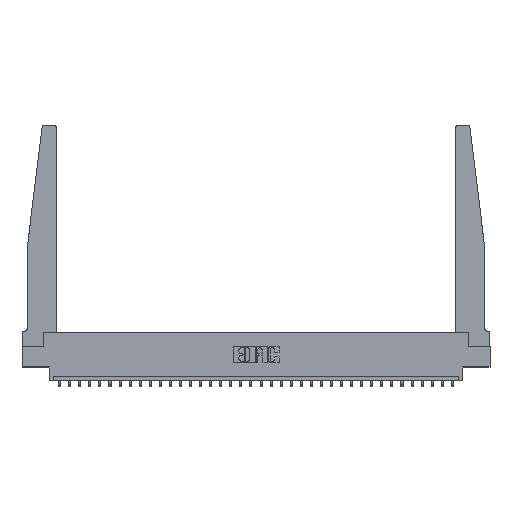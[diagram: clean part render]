
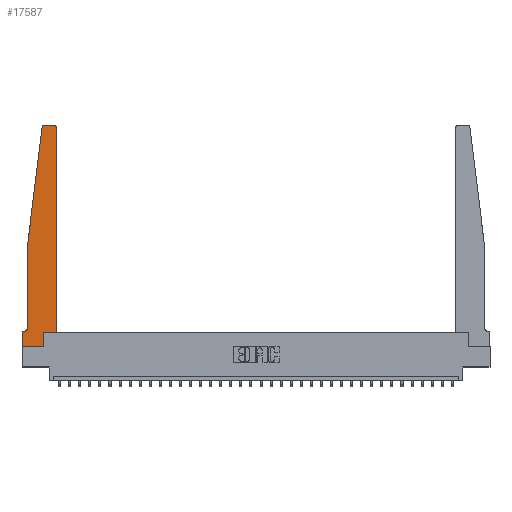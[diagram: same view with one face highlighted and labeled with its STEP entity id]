
A CAD part, top view. The second image highlights one B-rep face of the part: STEP entity #17587.
In plain terms, the highlighted planar face has unit normal (0, 0, 1).
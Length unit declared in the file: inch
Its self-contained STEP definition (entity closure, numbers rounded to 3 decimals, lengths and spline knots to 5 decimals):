
#184 = LINE ( 'NONE', #27953, #18059 ) ;
#449 = VERTEX_POINT ( 'NONE', #13266 ) ;
#829 = LINE ( 'NONE', #26259, #12484 ) ;
#838 = CARTESIAN_POINT ( 'NONE',  ( 0.065, 1.25, 0.37 ) ) ;
#891 = CARTESIAN_POINT ( 'NONE',  ( 0.015, 0.2375, 0.37 ) ) ;
#1064 = EDGE_CURVE ( 'NONE', #24890, #20575, #15991, .T. ) ;
#1639 = EDGE_CURVE ( 'NONE', #25553, #26862, #17793, .T. ) ;
#1851 = ORIENTED_EDGE ( 'NONE', *, *, #1064, .T. ) ;
#2342 = CARTESIAN_POINT ( 'NONE',  ( 0.015, 0.1875, 0.37 ) ) ;
#2371 = LINE ( 'NONE', #28194, #14041 ) ;
#2573 = DIRECTION ( 'NONE',  ( 1., 0., 0. ) ) ;
#2595 = CARTESIAN_POINT ( 'NONE',  ( 0., 0., 0.37 ) ) ;
#2944 = PLANE ( 'NONE',  #10477 ) ;
#3221 = DIRECTION ( 'NONE',  ( -1., 0., 0. ) ) ;
#3519 = VERTEX_POINT ( 'NONE', #17491 ) ;
#3600 = ORIENTED_EDGE ( 'NONE', *, *, #22285, .T. ) ;
#3821 = ORIENTED_EDGE ( 'NONE', *, *, #8251, .T. ) ;
#4082 = VECTOR ( 'NONE', #27996, 39.37008 ) ;
#4531 = LINE ( 'NONE', #6041, #16272 ) ;
#4697 = EDGE_CURVE ( 'NONE', #26949, #24890, #27327, .T. ) ;
#5114 = VERTEX_POINT ( 'NONE', #7011 ) ;
#5982 = DIRECTION ( 'NONE',  ( 0., 0., 1. ) ) ;
#6041 = CARTESIAN_POINT ( 'NONE',  ( 0.425, 0.18, 0.37 ) ) ;
#6273 = EDGE_CURVE ( 'NONE', #3519, #15491, #16355, .T. ) ;
#6381 = VERTEX_POINT ( 'NONE', #2595 ) ;
#6476 = CARTESIAN_POINT ( 'NONE',  ( 0.065, 0.2375, 0.37 ) ) ;
#6590 = ORIENTED_EDGE ( 'NONE', *, *, #24447, .T. ) ;
#6827 = AXIS2_PLACEMENT_3D ( 'NONE', #20009, #5982, #22331 ) ;
#7011 = CARTESIAN_POINT ( 'NONE',  ( 0.2605, 0., 0.37 ) ) ;
#8229 = ORIENTED_EDGE ( 'NONE', *, *, #28658, .T. ) ;
#8251 = EDGE_CURVE ( 'NONE', #5114, #449, #184, .T. ) ;
#8418 = DIRECTION ( 'NONE',  ( 0., 1., 0. ) ) ;
#8603 = ORIENTED_EDGE ( 'NONE', *, *, #10242, .T. ) ;
#8953 = CARTESIAN_POINT ( 'NONE',  ( 0., 0., 0.37 ) ) ;
#9014 = VECTOR ( 'NONE', #10866, 39.37008 ) ;
#9491 = CARTESIAN_POINT ( 'NONE',  ( 0., 0., 0.37 ) ) ;
#10206 = VERTEX_POINT ( 'NONE', #21589 ) ;
#10242 = EDGE_CURVE ( 'NONE', #15491, #10206, #16654, .T. ) ;
#10423 = EDGE_CURVE ( 'NONE', #19759, #25553, #4531, .T. ) ;
#10459 = CARTESIAN_POINT ( 'NONE',  ( 0.425, 2.72, 0.37 ) ) ;
#10477 = AXIS2_PLACEMENT_3D ( 'NONE', #26213, #12312, #28528 ) ;
#10866 = DIRECTION ( 'NONE',  ( -1., 0., 0. ) ) ;
#12312 = DIRECTION ( 'NONE',  ( 0., 0., 1. ) ) ;
#12484 = VECTOR ( 'NONE', #14592, 39.37008 ) ;
#13266 = CARTESIAN_POINT ( 'NONE',  ( 0.2605, 0.18, 0.37 ) ) ;
#13816 = DIRECTION ( 'NONE',  ( 0., 0., 1. ) ) ;
#14041 = VECTOR ( 'NONE', #18997, 39.37008 ) ;
#14592 = DIRECTION ( 'NONE',  ( 1., 0., 0. ) ) ;
#15175 = VECTOR ( 'NONE', #19484, 39.37008 ) ;
#15187 = VECTOR ( 'NONE', #2573, 39.37008 ) ;
#15491 = VERTEX_POINT ( 'NONE', #16072 ) ;
#15991 = LINE ( 'NONE', #22467, #9014 ) ;
#16072 = CARTESIAN_POINT ( 'NONE',  ( 0.24675, 2.72367, 0.37 ) ) ;
#16272 = VECTOR ( 'NONE', #8418, 39.37008 ) ;
#16355 = CIRCLE ( 'NONE', #20051, 0.03 ) ;
#16509 = LINE ( 'NONE', #25681, #4082 ) ;
#16654 = LINE ( 'NONE', #838, #15175 ) ;
#16792 = CARTESIAN_POINT ( 'NONE',  ( 0., 0.1875, 0.37 ) ) ;
#17212 = DIRECTION ( 'NONE',  ( 0., 0., -1. ) ) ;
#17491 = CARTESIAN_POINT ( 'NONE',  ( 0.27653, 2.75, 0.37 ) ) ;
#17587 = ADVANCED_FACE ( 'NONE', ( #18729 ), #2944, .T. ) ;
#17793 = CIRCLE ( 'NONE', #6827, 0.03 ) ;
#17976 = CARTESIAN_POINT ( 'NONE',  ( 0.395, 2.75, 0.37 ) ) ;
#18059 = VECTOR ( 'NONE', #25634, 39.37008 ) ;
#18097 = EDGE_CURVE ( 'NONE', #26862, #3519, #16509, .T. ) ;
#18729 = FACE_OUTER_BOUND ( 'NONE', #28588, .T. ) ;
#18997 = DIRECTION ( 'NONE',  ( 0., -1., 0. ) ) ;
#19314 = LINE ( 'NONE', #8953, #24001 ) ;
#19484 = DIRECTION ( 'NONE',  ( -0.122, -0.992, 0. ) ) ;
#19619 = ORIENTED_EDGE ( 'NONE', *, *, #18097, .T. ) ;
#19759 = VERTEX_POINT ( 'NONE', #24801 ) ;
#20009 = CARTESIAN_POINT ( 'NONE',  ( 0.395, 2.72, 0.37 ) ) ;
#20051 = AXIS2_PLACEMENT_3D ( 'NONE', #27708, #13816, #30029 ) ;
#20522 = ORIENTED_EDGE ( 'NONE', *, *, #4697, .T. ) ;
#20575 = VERTEX_POINT ( 'NONE', #16792 ) ;
#21589 = CARTESIAN_POINT ( 'NONE',  ( 0.065, 1.25, 0.37 ) ) ;
#21745 = ORIENTED_EDGE ( 'NONE', *, *, #6273, .T. ) ;
#22087 = LINE ( 'NONE', #9491, #15187 ) ;
#22285 = EDGE_CURVE ( 'NONE', #10206, #26949, #2371, .T. ) ;
#22331 = DIRECTION ( 'NONE',  ( 1., 0., 0. ) ) ;
#22352 = AXIS2_PLACEMENT_3D ( 'NONE', #891, #17212, #3221 ) ;
#22467 = CARTESIAN_POINT ( 'NONE',  ( 0.065, 0.1875, 0.37 ) ) ;
#24001 = VECTOR ( 'NONE', #27561, 39.37008 ) ;
#24447 = EDGE_CURVE ( 'NONE', #449, #19759, #829, .T. ) ;
#24801 = CARTESIAN_POINT ( 'NONE',  ( 0.425, 0.18, 0.37 ) ) ;
#24821 = ORIENTED_EDGE ( 'NONE', *, *, #10423, .T. ) ;
#24890 = VERTEX_POINT ( 'NONE', #2342 ) ;
#25553 = VERTEX_POINT ( 'NONE', #10459 ) ;
#25634 = DIRECTION ( 'NONE',  ( 0., 1., 0. ) ) ;
#25681 = CARTESIAN_POINT ( 'NONE',  ( 0.25, 2.75, 0.37 ) ) ;
#26213 = CARTESIAN_POINT ( 'NONE',  ( 0., 0.1875, 0.37 ) ) ;
#26259 = CARTESIAN_POINT ( 'NONE',  ( 0.425, 0.18, 0.37 ) ) ;
#26648 = ORIENTED_EDGE ( 'NONE', *, *, #26968, .T. ) ;
#26862 = VERTEX_POINT ( 'NONE', #17976 ) ;
#26949 = VERTEX_POINT ( 'NONE', #6476 ) ;
#26968 = EDGE_CURVE ( 'NONE', #20575, #6381, #19314, .T. ) ;
#27327 = CIRCLE ( 'NONE', #22352, 0.05 ) ;
#27561 = DIRECTION ( 'NONE',  ( 0., -1., 0. ) ) ;
#27708 = CARTESIAN_POINT ( 'NONE',  ( 0.27653, 2.72, 0.37 ) ) ;
#27728 = ORIENTED_EDGE ( 'NONE', *, *, #1639, .T. ) ;
#27953 = CARTESIAN_POINT ( 'NONE',  ( 0.2605, 0.18, 0.37 ) ) ;
#27996 = DIRECTION ( 'NONE',  ( -1., 0., 0. ) ) ;
#28194 = CARTESIAN_POINT ( 'NONE',  ( 0.065, 1.25, 0.37 ) ) ;
#28528 = DIRECTION ( 'NONE',  ( 1., 0., 0. ) ) ;
#28588 = EDGE_LOOP ( 'NONE', ( #19619, #21745, #8603, #3600, #20522, #1851, #26648, #8229, #3821, #6590, #24821, #27728 ) ) ;
#28658 = EDGE_CURVE ( 'NONE', #6381, #5114, #22087, .T. ) ;
#30029 = DIRECTION ( 'NONE',  ( 1., 0., 0. ) ) ;
